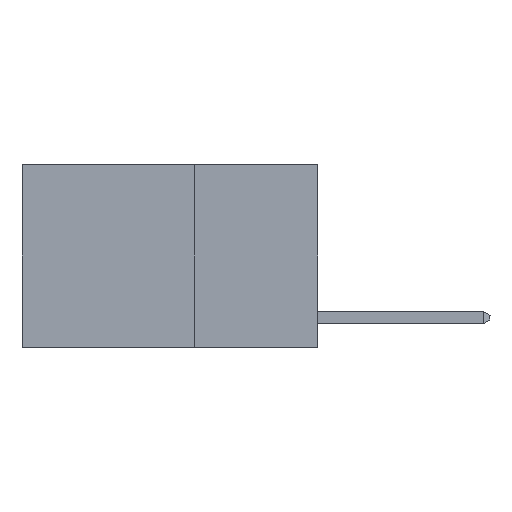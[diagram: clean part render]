
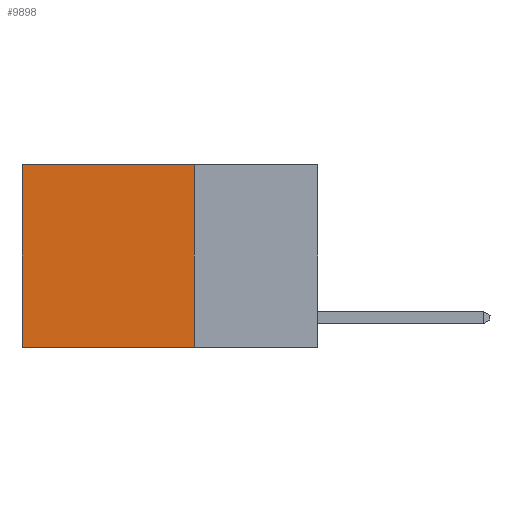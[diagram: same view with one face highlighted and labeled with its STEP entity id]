
A CAD part, left-side view. The second image highlights one B-rep face of the part: STEP entity #9898.
In plain terms, the highlighted planar face has unit normal (-1, 0, 0).
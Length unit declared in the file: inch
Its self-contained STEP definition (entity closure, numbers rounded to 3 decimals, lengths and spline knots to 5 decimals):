
#641 = VERTEX_POINT ( 'NONE', #14452 ) ;
#1674 = EDGE_CURVE ( 'NONE', #4172, #641, #17392, .T. ) ;
#1750 = LINE ( 'NONE', #15376, #11904 ) ;
#3709 = DIRECTION ( 'NONE',  ( 0., 0., -1. ) ) ;
#3930 = CARTESIAN_POINT ( 'NONE',  ( 0.2625, 0.25, -0.37 ) ) ;
#4172 = VERTEX_POINT ( 'NONE', #20731 ) ;
#5275 = VERTEX_POINT ( 'NONE', #12905 ) ;
#6577 = ORIENTED_EDGE ( 'NONE', *, *, #6951, .F. ) ;
#6743 = CARTESIAN_POINT ( 'NONE',  ( 0.2625, 0.25, 0. ) ) ;
#6951 = EDGE_CURVE ( 'NONE', #5275, #4172, #1750, .T. ) ;
#7743 = AXIS2_PLACEMENT_3D ( 'NONE', #6743, #17883, #27478 ) ;
#8680 = EDGE_CURVE ( 'NONE', #19115, #641, #29468, .T. ) ;
#9898 = ADVANCED_FACE ( 'NONE', ( #25131 ), #22647, .F. ) ;
#10074 = EDGE_CURVE ( 'NONE', #5275, #19115, #17369, .T. ) ;
#11297 = ORIENTED_EDGE ( 'NONE', *, *, #1674, .F. ) ;
#11904 = VECTOR ( 'NONE', #15069, 39.37008 ) ;
#12905 = CARTESIAN_POINT ( 'NONE',  ( 0.2625, 0.25, 0. ) ) ;
#14452 = CARTESIAN_POINT ( 'NONE',  ( 0.2625, 0.6, -0.37 ) ) ;
#15069 = DIRECTION ( 'NONE',  ( 0., 0., -1. ) ) ;
#15376 = CARTESIAN_POINT ( 'NONE',  ( 0.2625, 0.25, 0. ) ) ;
#16982 = ORIENTED_EDGE ( 'NONE', *, *, #8680, .T. ) ;
#17369 = LINE ( 'NONE', #29241, #23921 ) ;
#17392 = LINE ( 'NONE', #3930, #18091 ) ;
#17883 = DIRECTION ( 'NONE',  ( 1., 0., 0. ) ) ;
#18091 = VECTOR ( 'NONE', #19991, 39.37008 ) ;
#19115 = VERTEX_POINT ( 'NONE', #19625 ) ;
#19625 = CARTESIAN_POINT ( 'NONE',  ( 0.2625, 0.6, 0. ) ) ;
#19970 = DIRECTION ( 'NONE',  ( 0., 1., 0. ) ) ;
#19991 = DIRECTION ( 'NONE',  ( 0., 1., 0. ) ) ;
#20731 = CARTESIAN_POINT ( 'NONE',  ( 0.2625, 0.25, -0.37 ) ) ;
#21892 = EDGE_LOOP ( 'NONE', ( #16982, #11297, #6577, #25444 ) ) ;
#22647 = PLANE ( 'NONE',  #7743 ) ;
#23312 = VECTOR ( 'NONE', #3709, 39.37008 ) ;
#23921 = VECTOR ( 'NONE', #19970, 39.37008 ) ;
#24384 = CARTESIAN_POINT ( 'NONE',  ( 0.2625, 0.6, 0. ) ) ;
#25131 = FACE_OUTER_BOUND ( 'NONE', #21892, .T. ) ;
#25444 = ORIENTED_EDGE ( 'NONE', *, *, #10074, .T. ) ;
#27478 = DIRECTION ( 'NONE',  ( 0., 0., -1. ) ) ;
#29241 = CARTESIAN_POINT ( 'NONE',  ( 0.2625, 0.25, 0. ) ) ;
#29468 = LINE ( 'NONE', #24384, #23312 ) ;
